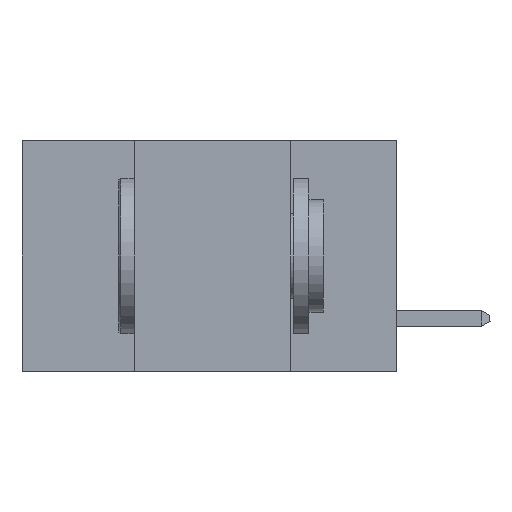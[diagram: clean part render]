
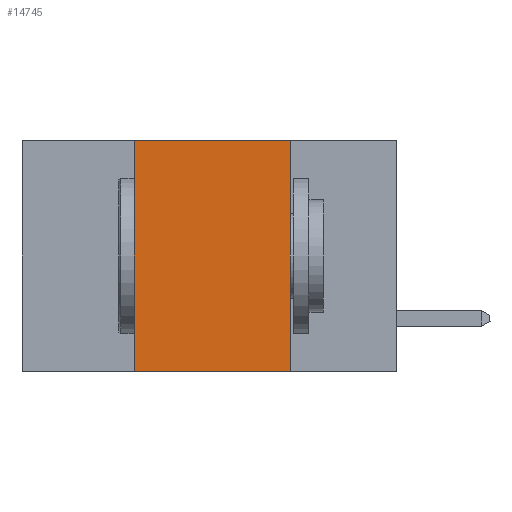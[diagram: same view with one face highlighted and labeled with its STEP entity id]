
A CAD part, left-side view. The second image highlights one B-rep face of the part: STEP entity #14745.
In plain terms, the highlighted planar face has unit normal (-1, 0, 0).
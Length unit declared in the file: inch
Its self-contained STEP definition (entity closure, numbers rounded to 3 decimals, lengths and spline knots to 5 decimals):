
#540 = CARTESIAN_POINT ( 'NONE',  ( 0., 0.42, 0. ) ) ;
#2134 = AXIS2_PLACEMENT_3D ( 'NONE', #2867, #16194, #7356 ) ;
#2280 = VERTEX_POINT ( 'NONE', #8494 ) ;
#2533 = ORIENTED_EDGE ( 'NONE', *, *, #7482, .F. ) ;
#2867 = CARTESIAN_POINT ( 'NONE',  ( 0., 0.6, 0. ) ) ;
#3853 = LINE ( 'NONE', #16068, #11412 ) ;
#4330 = PLANE ( 'NONE',  #2134 ) ;
#4395 = VECTOR ( 'NONE', #18467, 39.37008 ) ;
#4719 = FACE_OUTER_BOUND ( 'NONE', #13652, .T. ) ;
#5582 = CARTESIAN_POINT ( 'NONE',  ( 0., 0.42, -0.37 ) ) ;
#6471 = EDGE_CURVE ( 'NONE', #8789, #11483, #12817, .T. ) ;
#6739 = VECTOR ( 'NONE', #9309, 39.37008 ) ;
#7220 = CARTESIAN_POINT ( 'NONE',  ( 0., 0.17, 0. ) ) ;
#7356 = DIRECTION ( 'NONE',  ( 0., 0., -1. ) ) ;
#7482 = EDGE_CURVE ( 'NONE', #12892, #2280, #14157, .T. ) ;
#8126 = ORIENTED_EDGE ( 'NONE', *, *, #6471, .F. ) ;
#8494 = CARTESIAN_POINT ( 'NONE',  ( 0., 0.17, -0.37 ) ) ;
#8528 = DIRECTION ( 'NONE',  ( 0., -1., 0. ) ) ;
#8789 = VERTEX_POINT ( 'NONE', #5582 ) ;
#9309 = DIRECTION ( 'NONE',  ( 0., 0., -1. ) ) ;
#9444 = CARTESIAN_POINT ( 'NONE',  ( 0., 0.17, 0. ) ) ;
#11412 = VECTOR ( 'NONE', #17488, 39.37008 ) ;
#11483 = VERTEX_POINT ( 'NONE', #540 ) ;
#11682 = EDGE_CURVE ( 'NONE', #11483, #12892, #13762, .T. ) ;
#12558 = ORIENTED_EDGE ( 'NONE', *, *, #12850, .T. ) ;
#12817 = LINE ( 'NONE', #18876, #4395 ) ;
#12850 = EDGE_CURVE ( 'NONE', #8789, #2280, #3853, .T. ) ;
#12892 = VERTEX_POINT ( 'NONE', #7220 ) ;
#12930 = CARTESIAN_POINT ( 'NONE',  ( 0., 0.6, 0. ) ) ;
#13652 = EDGE_LOOP ( 'NONE', ( #2533, #15724, #8126, #12558 ) ) ;
#13762 = LINE ( 'NONE', #12930, #17145 ) ;
#14157 = LINE ( 'NONE', #9444, #6739 ) ;
#14745 = ADVANCED_FACE ( 'NONE', ( #4719 ), #4330, .F. ) ;
#15724 = ORIENTED_EDGE ( 'NONE', *, *, #11682, .F. ) ;
#16068 = CARTESIAN_POINT ( 'NONE',  ( 0., 0.6, -0.37 ) ) ;
#16194 = DIRECTION ( 'NONE',  ( 1., 0., 0. ) ) ;
#17145 = VECTOR ( 'NONE', #8528, 39.37008 ) ;
#17488 = DIRECTION ( 'NONE',  ( 0., -1., 0. ) ) ;
#18467 = DIRECTION ( 'NONE',  ( 0., 0., 1. ) ) ;
#18876 = CARTESIAN_POINT ( 'NONE',  ( 0., 0.42, 0. ) ) ;
